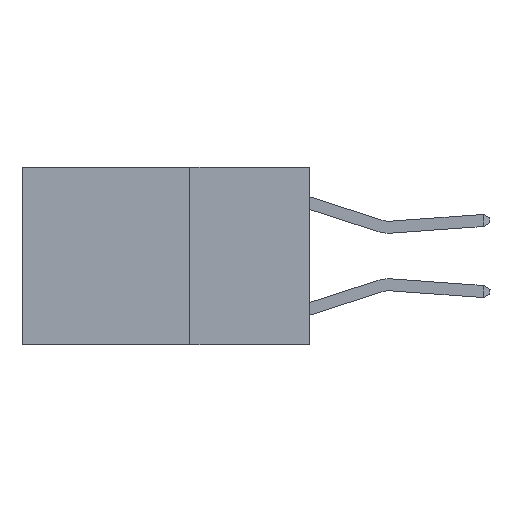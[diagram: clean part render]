
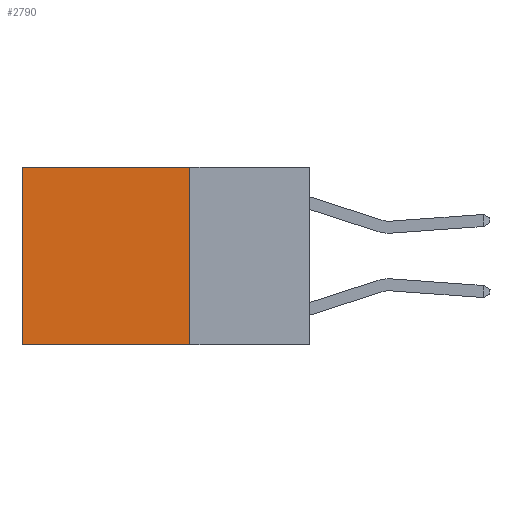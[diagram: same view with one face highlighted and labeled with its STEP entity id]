
A CAD part, left-side view. The second image highlights one B-rep face of the part: STEP entity #2790.
In plain terms, the highlighted planar face has unit normal (-1, 0, 0).
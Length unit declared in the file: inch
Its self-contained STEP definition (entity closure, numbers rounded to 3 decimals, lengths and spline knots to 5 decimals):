
#593 = EDGE_CURVE ( 'NONE', #7554, #6414, #6272, .T. ) ;
#1373 = CARTESIAN_POINT ( 'NONE',  ( 0.2625, 0.25, -0.37 ) ) ;
#1447 = LINE ( 'NONE', #8663, #10832 ) ;
#1747 = EDGE_LOOP ( 'NONE', ( #4655, #4394, #6717, #5860 ) ) ;
#2201 = CARTESIAN_POINT ( 'NONE',  ( 0.2625, 0.6, 0. ) ) ;
#2379 = CARTESIAN_POINT ( 'NONE',  ( 0.2625, 0.6, -0.37 ) ) ;
#2392 = CARTESIAN_POINT ( 'NONE',  ( 0.2625, 0.25, 0. ) ) ;
#2647 = CARTESIAN_POINT ( 'NONE',  ( 0.2625, 0.25, 0. ) ) ;
#2701 = AXIS2_PLACEMENT_3D ( 'NONE', #2392, #10585, #5158 ) ;
#2790 = ADVANCED_FACE ( 'NONE', ( #10189 ), #11456, .F. ) ;
#2818 = CARTESIAN_POINT ( 'NONE',  ( 0.2625, 0.25, 0. ) ) ;
#3220 = DIRECTION ( 'NONE',  ( 0., 1., 0. ) ) ;
#3395 = EDGE_CURVE ( 'NONE', #5839, #6414, #11152, .T. ) ;
#4328 = VECTOR ( 'NONE', #8112, 39.37008 ) ;
#4394 = ORIENTED_EDGE ( 'NONE', *, *, #3395, .F. ) ;
#4609 = LINE ( 'NONE', #2647, #4328 ) ;
#4655 = ORIENTED_EDGE ( 'NONE', *, *, #593, .T. ) ;
#5158 = DIRECTION ( 'NONE',  ( 0., 0., -1. ) ) ;
#5378 = EDGE_CURVE ( 'NONE', #7748, #5839, #4609, .T. ) ;
#5839 = VERTEX_POINT ( 'NONE', #10555 ) ;
#5860 = ORIENTED_EDGE ( 'NONE', *, *, #8045, .T. ) ;
#6217 = DIRECTION ( 'NONE',  ( 0., 0., -1. ) ) ;
#6272 = LINE ( 'NONE', #7096, #9963 ) ;
#6414 = VERTEX_POINT ( 'NONE', #2379 ) ;
#6717 = ORIENTED_EDGE ( 'NONE', *, *, #5378, .F. ) ;
#6889 = DIRECTION ( 'NONE',  ( 0., 1., 0. ) ) ;
#7096 = CARTESIAN_POINT ( 'NONE',  ( 0.2625, 0.6, 0. ) ) ;
#7554 = VERTEX_POINT ( 'NONE', #2201 ) ;
#7748 = VERTEX_POINT ( 'NONE', #2818 ) ;
#8045 = EDGE_CURVE ( 'NONE', #7748, #7554, #1447, .T. ) ;
#8112 = DIRECTION ( 'NONE',  ( 0., 0., -1. ) ) ;
#8663 = CARTESIAN_POINT ( 'NONE',  ( 0.2625, 0.25, 0. ) ) ;
#8760 = VECTOR ( 'NONE', #3220, 39.37008 ) ;
#9963 = VECTOR ( 'NONE', #6217, 39.37008 ) ;
#10189 = FACE_OUTER_BOUND ( 'NONE', #1747, .T. ) ;
#10555 = CARTESIAN_POINT ( 'NONE',  ( 0.2625, 0.25, -0.37 ) ) ;
#10585 = DIRECTION ( 'NONE',  ( 1., 0., 0. ) ) ;
#10832 = VECTOR ( 'NONE', #6889, 39.37008 ) ;
#11152 = LINE ( 'NONE', #1373, #8760 ) ;
#11456 = PLANE ( 'NONE',  #2701 ) ;
